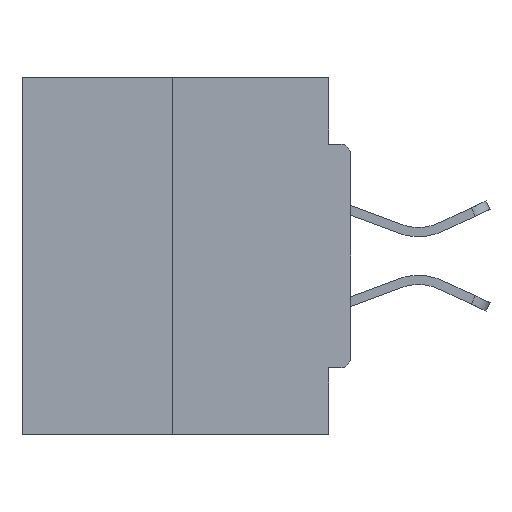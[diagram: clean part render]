
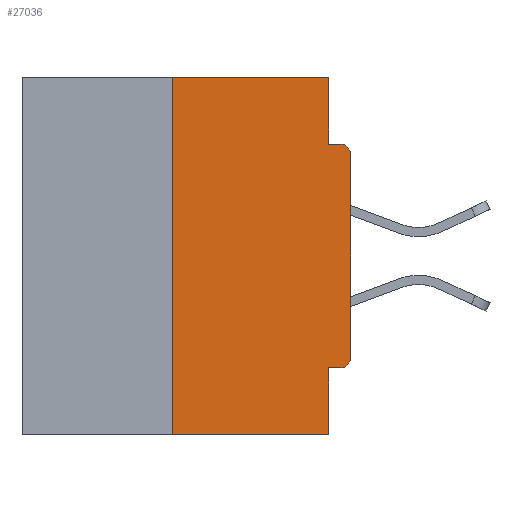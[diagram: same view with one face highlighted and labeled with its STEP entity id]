
A CAD part, left-side view. The second image highlights one B-rep face of the part: STEP entity #27036.
In plain terms, the highlighted planar face has unit normal (-1, 0, 0).
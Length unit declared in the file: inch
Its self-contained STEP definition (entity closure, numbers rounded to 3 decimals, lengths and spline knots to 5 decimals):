
#804 = AXIS2_PLACEMENT_3D ( 'NONE', #9015, #34401, #23189 ) ;
#1199 = EDGE_CURVE ( 'NONE', #15231, #6709, #33023, .T. ) ;
#1397 = VERTEX_POINT ( 'NONE', #35077 ) ;
#2077 = CARTESIAN_POINT ( 'NONE',  ( 0., 0.031, -0.5 ) ) ;
#2194 = ORIENTED_EDGE ( 'NONE', *, *, #1199, .T. ) ;
#2300 = VERTEX_POINT ( 'NONE', #3014 ) ;
#2303 = EDGE_LOOP ( 'NONE', ( #9791, #15572, #21148, #23819, #35499, #19268, #2194, #38629, #31670, #6354 ) ) ;
#3014 = CARTESIAN_POINT ( 'NONE',  ( 0., 0.25, -0.5 ) ) ;
#6023 = DIRECTION ( 'NONE',  ( 0., -1., 0. ) ) ;
#6280 = VECTOR ( 'NONE', #11817, 39.37008 ) ;
#6354 = ORIENTED_EDGE ( 'NONE', *, *, #44522, .F. ) ;
#6375 = VECTOR ( 'NONE', #27711, 39.37008 ) ;
#6709 = VERTEX_POINT ( 'NONE', #16810 ) ;
#6737 = DIRECTION ( 'NONE',  ( 0., -1., 0. ) ) ;
#6973 = CARTESIAN_POINT ( 'NONE',  ( 0., 0.25, 0. ) ) ;
#7515 = EDGE_CURVE ( 'NONE', #29404, #34851, #39702, .T. ) ;
#9015 = CARTESIAN_POINT ( 'NONE',  ( 0., 0.015, -0.3915 ) ) ;
#9306 = EDGE_CURVE ( 'NONE', #29404, #15231, #44779, .T. ) ;
#9631 = VERTEX_POINT ( 'NONE', #40165 ) ;
#9791 = ORIENTED_EDGE ( 'NONE', *, *, #18756, .F. ) ;
#9901 = FACE_OUTER_BOUND ( 'NONE', #2303, .T. ) ;
#10153 = PLANE ( 'NONE',  #33882 ) ;
#11162 = CARTESIAN_POINT ( 'NONE',  ( 0., 0.015, -0.1085 ) ) ;
#11676 = CARTESIAN_POINT ( 'NONE',  ( 0., 0.015, -0.4065 ) ) ;
#11817 = DIRECTION ( 'NONE',  ( 0., 0., 1. ) ) ;
#12119 = AXIS2_PLACEMENT_3D ( 'NONE', #11162, #36112, #36351 ) ;
#13027 = LINE ( 'NONE', #41499, #30020 ) ;
#13031 = CARTESIAN_POINT ( 'NONE',  ( 0., 0.46, -0.5 ) ) ;
#13505 = CARTESIAN_POINT ( 'NONE',  ( 0., 0., -0.0935 ) ) ;
#15231 = VERTEX_POINT ( 'NONE', #44945 ) ;
#15392 = CARTESIAN_POINT ( 'NONE',  ( 0., 0.031, -0.4065 ) ) ;
#15477 = VERTEX_POINT ( 'NONE', #39063 ) ;
#15572 = ORIENTED_EDGE ( 'NONE', *, *, #38427, .F. ) ;
#16810 = CARTESIAN_POINT ( 'NONE',  ( 0., 0., -0.1085 ) ) ;
#17206 = CARTESIAN_POINT ( 'NONE',  ( 0., 0.031, 0. ) ) ;
#18756 = EDGE_CURVE ( 'NONE', #15477, #30945, #13027, .T. ) ;
#19268 = ORIENTED_EDGE ( 'NONE', *, *, #9306, .T. ) ;
#19894 = CARTESIAN_POINT ( 'NONE',  ( 0., 0.031, 0. ) ) ;
#21148 = ORIENTED_EDGE ( 'NONE', *, *, #23666, .T. ) ;
#21715 = DIRECTION ( 'NONE',  ( 0., 1., 0. ) ) ;
#22548 = VECTOR ( 'NONE', #37755, 39.37008 ) ;
#22979 = VERTEX_POINT ( 'NONE', #23814 ) ;
#23189 = DIRECTION ( 'NONE',  ( 0., 0., -1. ) ) ;
#23265 = CIRCLE ( 'NONE', #12119, 0.015 ) ;
#23666 = EDGE_CURVE ( 'NONE', #2300, #22979, #45252, .T. ) ;
#23814 = CARTESIAN_POINT ( 'NONE',  ( 0., 0.031, -0.5 ) ) ;
#23819 = ORIENTED_EDGE ( 'NONE', *, *, #33104, .F. ) ;
#24332 = CARTESIAN_POINT ( 'NONE',  ( 0., 0.46, 0. ) ) ;
#24444 = LINE ( 'NONE', #13505, #29316 ) ;
#25882 = DIRECTION ( 'NONE',  ( 0., 0., -1. ) ) ;
#27036 = ADVANCED_FACE ( 'NONE', ( #9901 ), #10153, .F. ) ;
#27711 = DIRECTION ( 'NONE',  ( 0., 0., 1. ) ) ;
#29316 = VECTOR ( 'NONE', #6737, 39.37008 ) ;
#29404 = VERTEX_POINT ( 'NONE', #11676 ) ;
#29611 = LINE ( 'NONE', #2077, #29906 ) ;
#29906 = VECTOR ( 'NONE', #25882, 39.37008 ) ;
#29913 = VECTOR ( 'NONE', #30493, 39.37008 ) ;
#30020 = VECTOR ( 'NONE', #6023, 39.37008 ) ;
#30410 = DIRECTION ( 'NONE',  ( 1., 0., 0. ) ) ;
#30493 = DIRECTION ( 'NONE',  ( 0., -1., 0. ) ) ;
#30945 = VERTEX_POINT ( 'NONE', #19894 ) ;
#31670 = ORIENTED_EDGE ( 'NONE', *, *, #45449, .F. ) ;
#33023 = LINE ( 'NONE', #43796, #6280 ) ;
#33104 = EDGE_CURVE ( 'NONE', #34851, #22979, #29611, .T. ) ;
#33882 = AXIS2_PLACEMENT_3D ( 'NONE', #24332, #30410, #35536 ) ;
#34401 = DIRECTION ( 'NONE',  ( -1., 0., 0. ) ) ;
#34851 = VERTEX_POINT ( 'NONE', #15392 ) ;
#34949 = LINE ( 'NONE', #17206, #22548 ) ;
#35077 = CARTESIAN_POINT ( 'NONE',  ( 0., 0.031, -0.0935 ) ) ;
#35499 = ORIENTED_EDGE ( 'NONE', *, *, #7515, .F. ) ;
#35536 = DIRECTION ( 'NONE',  ( 0., 0., -1. ) ) ;
#36112 = DIRECTION ( 'NONE',  ( -1., 0., 0. ) ) ;
#36351 = DIRECTION ( 'NONE',  ( 0., 0., -1. ) ) ;
#37755 = DIRECTION ( 'NONE',  ( 0., 0., -1. ) ) ;
#38427 = EDGE_CURVE ( 'NONE', #2300, #15477, #38901, .T. ) ;
#38629 = ORIENTED_EDGE ( 'NONE', *, *, #45611, .T. ) ;
#38901 = LINE ( 'NONE', #6973, #6375 ) ;
#39063 = CARTESIAN_POINT ( 'NONE',  ( 0., 0.25, 0. ) ) ;
#39702 = LINE ( 'NONE', #39952, #42547 ) ;
#39952 = CARTESIAN_POINT ( 'NONE',  ( 0., 0., -0.4065 ) ) ;
#40165 = CARTESIAN_POINT ( 'NONE',  ( 0., 0.015, -0.0935 ) ) ;
#41499 = CARTESIAN_POINT ( 'NONE',  ( 0., 0.46, 0. ) ) ;
#42547 = VECTOR ( 'NONE', #21715, 39.37008 ) ;
#43796 = CARTESIAN_POINT ( 'NONE',  ( 0., 0., 0. ) ) ;
#44522 = EDGE_CURVE ( 'NONE', #30945, #1397, #34949, .T. ) ;
#44779 = CIRCLE ( 'NONE', #804, 0.015 ) ;
#44945 = CARTESIAN_POINT ( 'NONE',  ( 0., 0., -0.3915 ) ) ;
#45252 = LINE ( 'NONE', #13031, #29913 ) ;
#45449 = EDGE_CURVE ( 'NONE', #1397, #9631, #24444, .T. ) ;
#45611 = EDGE_CURVE ( 'NONE', #6709, #9631, #23265, .T. ) ;
